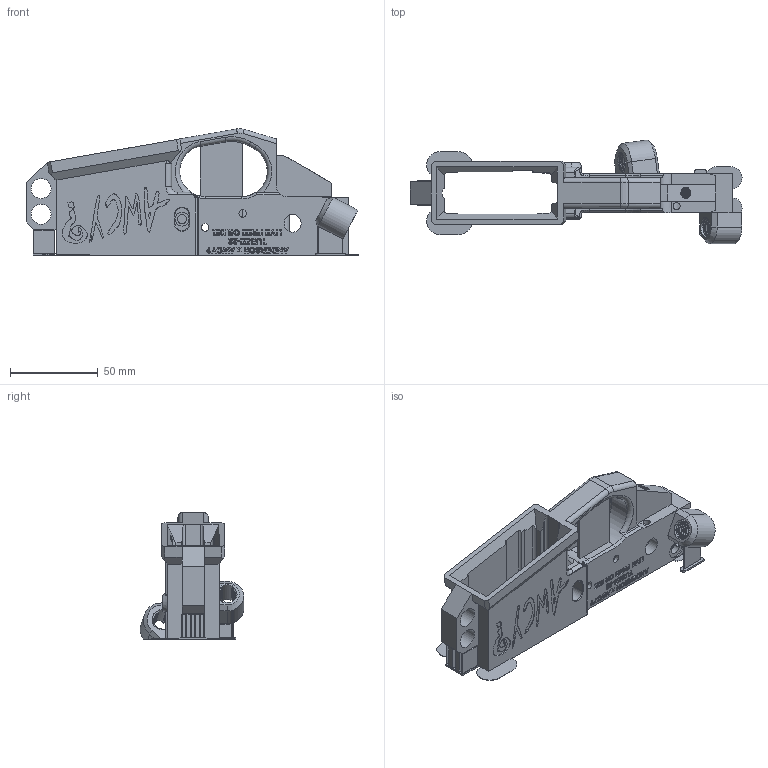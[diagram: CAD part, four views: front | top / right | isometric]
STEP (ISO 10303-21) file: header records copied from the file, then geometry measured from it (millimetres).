
FILE_DESCRIPTION(/* description */ (''),/* implementation_level */ '2;1');
FILE_NAME(/* name */ 'Tubee-22 Lower FINAL.step',/* time_stamp */ '2021-06-23T15:47:43-04:00',/* author */ (''),/* organization */ (''),/* preprocessor_version */ 'ST-DEVELOPER v18.1',/* originating_system */ 'Autodesk Translation Framework v10.9.0.1377',/* authorisation */ '');
FILE_SCHEMA (('AUTOMOTIVE_DESIGN { 1 0 10303 214 3 1 1 }'));
Products named in the file (6): Tubee-22; AR22 v11.step; Lower, Core; AR22 (v11~recovered)-38.step; AR22 (v11~recovered)-39.step; AR22 (v11~recovered)-40.step
Assembly tree (5 placements, depth 3):
  Tubee-22
    AR22 v11.step
      Lower, Core
      AR22 (v11~recovered)-38.step
      AR22 (v11~recovered)-39.step
      AR22 (v11~recovered)-40.step
Bounding box: 189.67 x 59.15 x 72.31 mm (x, y, z)
Volume: 99955.2 mm3; surface area: 70838.7 mm2
Topology: 4 solids, 4 shells, 2140 faces, 6053 edges, 4003 vertices
Faces by surface type: bspline 941, plane 915, cylinder 251, torus 17, cone 14, sphere 2
Full cylindrical faces by diameter (mm): 4.064 x1, 5.182 x1, 5.537 x21, 6.519 x22, 7.925 x1, 11.113 x1, 11.43 x2
Entity records: 113472 total; most frequent: CARTESIAN_POINT 64556, ORIENTED_EDGE 12104, DIRECTION 7009, EDGE_CURVE 6052, VERTEX_POINT 4003, LINE 3571, VECTOR 3571, EDGE_LOOP 2263
